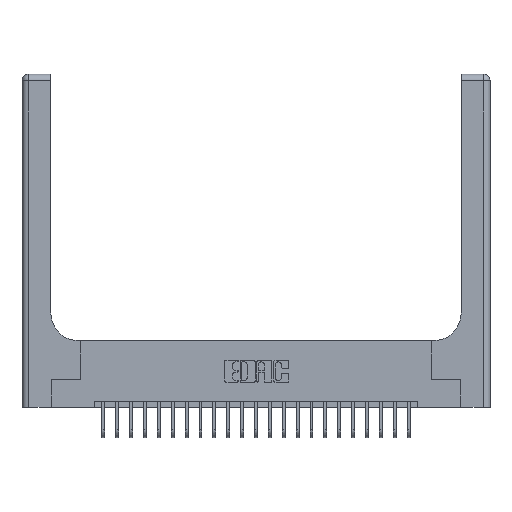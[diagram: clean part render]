
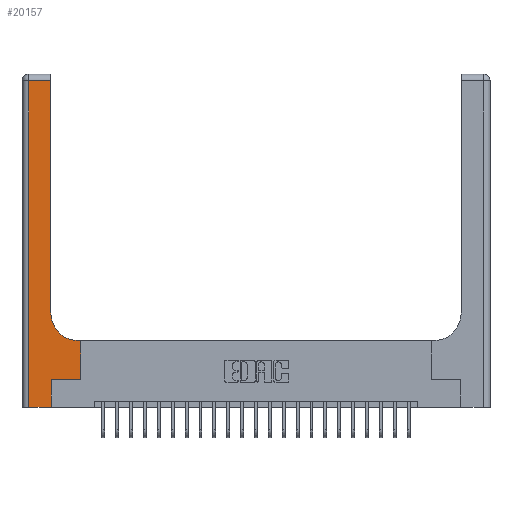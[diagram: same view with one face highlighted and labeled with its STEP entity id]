
A CAD part, top view. The second image highlights one B-rep face of the part: STEP entity #20157.
In plain terms, the highlighted planar face has unit normal (0, 0, 1).
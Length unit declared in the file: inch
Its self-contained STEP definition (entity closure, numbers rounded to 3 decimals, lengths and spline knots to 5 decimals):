
#344 = LINE ( 'NONE', #10399, #9901 ) ;
#1117 = ORIENTED_EDGE ( 'NONE', *, *, #16772, .T. ) ;
#1160 = DIRECTION ( 'NONE',  ( -1., 0., 0. ) ) ;
#1620 = ORIENTED_EDGE ( 'NONE', *, *, #11652, .T. ) ;
#2293 = CARTESIAN_POINT ( 'NONE',  ( 0.06, 3., 0.37 ) ) ;
#2722 = CARTESIAN_POINT ( 'NONE',  ( 0.265, 0.25, 0.37 ) ) ;
#2758 = EDGE_CURVE ( 'NONE', #10954, #21856, #344, .T. ) ;
#3072 = VECTOR ( 'NONE', #8291, 39.37008 ) ;
#3334 = VERTEX_POINT ( 'NONE', #24168 ) ;
#3948 = EDGE_CURVE ( 'NONE', #4833, #4073, #19104, .T. ) ;
#4073 = VERTEX_POINT ( 'NONE', #5773 ) ;
#4454 = CARTESIAN_POINT ( 'NONE',  ( 0.26, 3., 0.37 ) ) ;
#4739 = DIRECTION ( 'NONE',  ( 0., -1., 0. ) ) ;
#4833 = VERTEX_POINT ( 'NONE', #21230 ) ;
#5252 = ORIENTED_EDGE ( 'NONE', *, *, #6989, .T. ) ;
#5299 = ORIENTED_EDGE ( 'NONE', *, *, #21787, .T. ) ;
#5457 = CARTESIAN_POINT ( 'NONE',  ( 0., 3., 0.37 ) ) ;
#5620 = PLANE ( 'NONE',  #11638 ) ;
#5773 = CARTESIAN_POINT ( 'NONE',  ( 0.51, 0.6, 0.37 ) ) ;
#5928 = VERTEX_POINT ( 'NONE', #17546 ) ;
#6075 = ORIENTED_EDGE ( 'NONE', *, *, #2758, .T. ) ;
#6478 = EDGE_CURVE ( 'NONE', #8746, #21471, #11649, .T. ) ;
#6989 = EDGE_CURVE ( 'NONE', #4073, #5928, #15494, .T. ) ;
#7841 = CARTESIAN_POINT ( 'NONE',  ( 0.06, 0., 0.37 ) ) ;
#7962 = CARTESIAN_POINT ( 'NONE',  ( 0.51, 0.85, 0.37 ) ) ;
#8019 = EDGE_LOOP ( 'NONE', ( #20019, #19004, #22164, #1117, #5299, #6075, #1620, #17651, #5252 ) ) ;
#8291 = DIRECTION ( 'NONE',  ( 0., 1., 0. ) ) ;
#8365 = VECTOR ( 'NONE', #4739, 39.37008 ) ;
#8369 = CARTESIAN_POINT ( 'NONE',  ( 0.528, 0.25, 0.37 ) ) ;
#8746 = VERTEX_POINT ( 'NONE', #18143 ) ;
#9402 = CARTESIAN_POINT ( 'NONE',  ( 0., 0., 0.37 ) ) ;
#9747 = VERTEX_POINT ( 'NONE', #17426 ) ;
#9901 = VECTOR ( 'NONE', #23495, 39.37008 ) ;
#9998 = VECTOR ( 'NONE', #14850, 39.37008 ) ;
#10398 = DIRECTION ( 'NONE',  ( 1., 0., 0. ) ) ;
#10399 = CARTESIAN_POINT ( 'NONE',  ( 0.265, 0.25, 0.37 ) ) ;
#10792 = CARTESIAN_POINT ( 'NONE',  ( 0.528, 0.25, 0.37 ) ) ;
#10842 = DIRECTION ( 'NONE',  ( -1., 0., 0. ) ) ;
#10954 = VERTEX_POINT ( 'NONE', #2722 ) ;
#11414 = DIRECTION ( 'NONE',  ( -1., 0., 0. ) ) ;
#11638 = AXIS2_PLACEMENT_3D ( 'NONE', #5457, #18880, #11414 ) ;
#11649 = LINE ( 'NONE', #2293, #8365 ) ;
#11652 = EDGE_CURVE ( 'NONE', #21856, #4833, #17062, .T. ) ;
#11768 = LINE ( 'NONE', #14932, #9998 ) ;
#12684 = VECTOR ( 'NONE', #10842, 39.37008 ) ;
#13222 = DIRECTION ( 'NONE',  ( 1., 0., 0. ) ) ;
#13747 = VECTOR ( 'NONE', #15646, 39.37008 ) ;
#14850 = DIRECTION ( 'NONE',  ( 0., 1., 0. ) ) ;
#14932 = CARTESIAN_POINT ( 'NONE',  ( 0.265, 0., 0.37 ) ) ;
#15043 = LINE ( 'NONE', #23972, #12684 ) ;
#15494 = CIRCLE ( 'NONE', #17081, 0.25 ) ;
#15646 = DIRECTION ( 'NONE',  ( 0., 1., 0. ) ) ;
#15694 = LINE ( 'NONE', #9402, #20433 ) ;
#16772 = EDGE_CURVE ( 'NONE', #21471, #9747, #15694, .T. ) ;
#17062 = LINE ( 'NONE', #8369, #3072 ) ;
#17081 = AXIS2_PLACEMENT_3D ( 'NONE', #7962, #21447, #10398 ) ;
#17426 = CARTESIAN_POINT ( 'NONE',  ( 0.265, 0., 0.37 ) ) ;
#17546 = CARTESIAN_POINT ( 'NONE',  ( 0.26, 0.85, 0.37 ) ) ;
#17605 = LINE ( 'NONE', #4454, #13747 ) ;
#17651 = ORIENTED_EDGE ( 'NONE', *, *, #3948, .T. ) ;
#17824 = EDGE_CURVE ( 'NONE', #3334, #8746, #15043, .T. ) ;
#18143 = CARTESIAN_POINT ( 'NONE',  ( 0.06, 2.94, 0.37 ) ) ;
#18880 = DIRECTION ( 'NONE',  ( 0., 0., -1. ) ) ;
#19004 = ORIENTED_EDGE ( 'NONE', *, *, #17824, .T. ) ;
#19104 = LINE ( 'NONE', #23599, #19688 ) ;
#19688 = VECTOR ( 'NONE', #1160, 39.37008 ) ;
#20019 = ORIENTED_EDGE ( 'NONE', *, *, #24148, .T. ) ;
#20157 = ADVANCED_FACE ( 'NONE', ( #23071 ), #5620, .F. ) ;
#20433 = VECTOR ( 'NONE', #13222, 39.37008 ) ;
#21230 = CARTESIAN_POINT ( 'NONE',  ( 0.528, 0.6, 0.37 ) ) ;
#21447 = DIRECTION ( 'NONE',  ( 0., 0., -1. ) ) ;
#21471 = VERTEX_POINT ( 'NONE', #7841 ) ;
#21787 = EDGE_CURVE ( 'NONE', #9747, #10954, #11768, .T. ) ;
#21856 = VERTEX_POINT ( 'NONE', #10792 ) ;
#22164 = ORIENTED_EDGE ( 'NONE', *, *, #6478, .T. ) ;
#23071 = FACE_OUTER_BOUND ( 'NONE', #8019, .T. ) ;
#23495 = DIRECTION ( 'NONE',  ( 1., 0., 0. ) ) ;
#23599 = CARTESIAN_POINT ( 'NONE',  ( 0.26, 0.6, 0.37 ) ) ;
#23972 = CARTESIAN_POINT ( 'NONE',  ( 0., 2.94, 0.37 ) ) ;
#24148 = EDGE_CURVE ( 'NONE', #5928, #3334, #17605, .T. ) ;
#24168 = CARTESIAN_POINT ( 'NONE',  ( 0.26, 2.94, 0.37 ) ) ;
